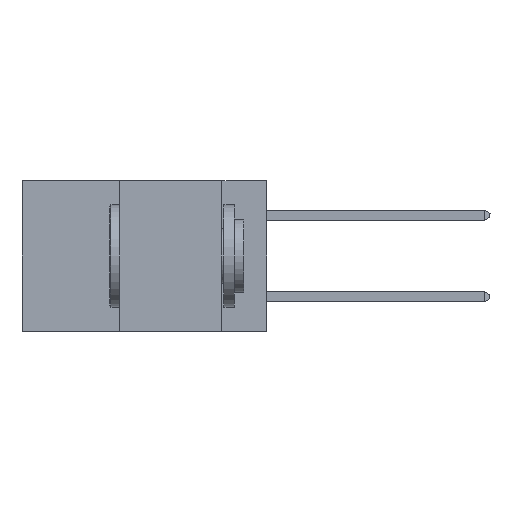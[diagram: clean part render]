
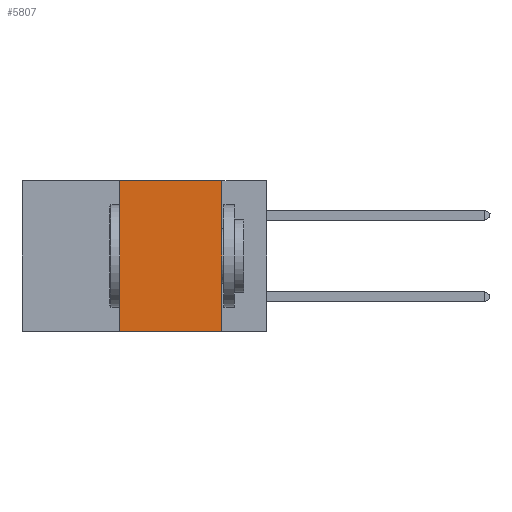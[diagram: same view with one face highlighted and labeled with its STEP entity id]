
A CAD part, left-side view. The second image highlights one B-rep face of the part: STEP entity #5807.
In plain terms, the highlighted planar face has unit normal (-1, 0, 0).
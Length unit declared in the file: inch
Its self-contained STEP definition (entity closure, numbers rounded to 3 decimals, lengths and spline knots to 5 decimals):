
#25 = LINE ( 'NONE', #12435, #16133 ) ;
#283 = CARTESIAN_POINT ( 'NONE',  ( 0., 0.36, 0. ) ) ;
#1294 = DIRECTION ( 'NONE',  ( 1., 0., 0. ) ) ;
#1740 = EDGE_CURVE ( 'NONE', #19327, #15040, #20211, .T. ) ;
#3448 = ORIENTED_EDGE ( 'NONE', *, *, #9277, .T. ) ;
#3782 = ORIENTED_EDGE ( 'NONE', *, *, #6884, .F. ) ;
#4290 = EDGE_CURVE ( 'NONE', #15040, #27127, #19987, .T. ) ;
#5807 = ADVANCED_FACE ( 'NONE', ( #20886 ), #7544, .F. ) ;
#6884 = EDGE_CURVE ( 'NONE', #27127, #9302, #15560, .T. ) ;
#7544 = PLANE ( 'NONE',  #19601 ) ;
#7714 = ORIENTED_EDGE ( 'NONE', *, *, #1740, .F. ) ;
#8020 = CARTESIAN_POINT ( 'NONE',  ( 0., 0.11, 0. ) ) ;
#8407 = VECTOR ( 'NONE', #10236, 39.37008 ) ;
#9277 = EDGE_CURVE ( 'NONE', #19327, #9302, #25, .T. ) ;
#9302 = VERTEX_POINT ( 'NONE', #14633 ) ;
#9993 = ORIENTED_EDGE ( 'NONE', *, *, #4290, .F. ) ;
#10001 = VECTOR ( 'NONE', #26113, 39.37008 ) ;
#10236 = DIRECTION ( 'NONE',  ( 0., 0., 1. ) ) ;
#10910 = CARTESIAN_POINT ( 'NONE',  ( 0., 0.6, 0. ) ) ;
#12435 = CARTESIAN_POINT ( 'NONE',  ( 0., 0.6, -0.37 ) ) ;
#13856 = CARTESIAN_POINT ( 'NONE',  ( 0., 0.6, 0. ) ) ;
#14633 = CARTESIAN_POINT ( 'NONE',  ( 0., 0.11, -0.37 ) ) ;
#15040 = VERTEX_POINT ( 'NONE', #283 ) ;
#15560 = LINE ( 'NONE', #21822, #10001 ) ;
#15960 = DIRECTION ( 'NONE',  ( 0., 0., -1. ) ) ;
#16133 = VECTOR ( 'NONE', #27197, 39.37008 ) ;
#16547 = CARTESIAN_POINT ( 'NONE',  ( 0., 0.36, -0.37 ) ) ;
#19327 = VERTEX_POINT ( 'NONE', #16547 ) ;
#19601 = AXIS2_PLACEMENT_3D ( 'NONE', #13856, #1294, #15960 ) ;
#19987 = LINE ( 'NONE', #10910, #26302 ) ;
#20211 = LINE ( 'NONE', #22826, #8407 ) ;
#20886 = FACE_OUTER_BOUND ( 'NONE', #24460, .T. ) ;
#21822 = CARTESIAN_POINT ( 'NONE',  ( 0., 0.11, 0. ) ) ;
#22826 = CARTESIAN_POINT ( 'NONE',  ( 0., 0.36, 0. ) ) ;
#23504 = DIRECTION ( 'NONE',  ( 0., -1., 0. ) ) ;
#24460 = EDGE_LOOP ( 'NONE', ( #3782, #9993, #7714, #3448 ) ) ;
#26113 = DIRECTION ( 'NONE',  ( 0., 0., -1. ) ) ;
#26302 = VECTOR ( 'NONE', #23504, 39.37008 ) ;
#27127 = VERTEX_POINT ( 'NONE', #8020 ) ;
#27197 = DIRECTION ( 'NONE',  ( 0., -1., 0. ) ) ;
